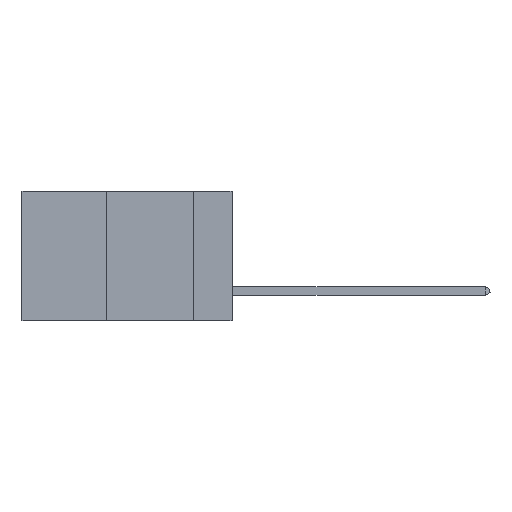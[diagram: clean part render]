
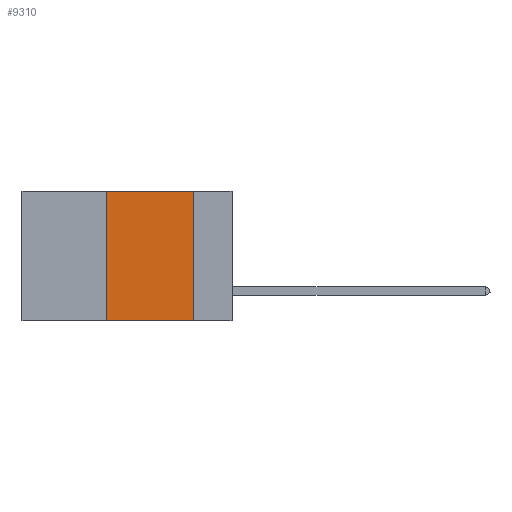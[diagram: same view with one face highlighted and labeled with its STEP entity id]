
A CAD part, left-side view. The second image highlights one B-rep face of the part: STEP entity #9310.
In plain terms, the highlighted planar face has unit normal (-1, 0, 0).
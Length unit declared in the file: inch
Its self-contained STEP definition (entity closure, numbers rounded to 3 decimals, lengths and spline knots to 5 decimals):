
#236 = DIRECTION ( 'NONE',  ( 1., 0., 0. ) ) ;
#335 = AXIS2_PLACEMENT_3D ( 'NONE', #10226, #236, #2248 ) ;
#501 = VERTEX_POINT ( 'NONE', #17729 ) ;
#902 = CARTESIAN_POINT ( 'NONE',  ( 0., 0.11, -0.37 ) ) ;
#1145 = CARTESIAN_POINT ( 'NONE',  ( 0., 0.36, -0.37 ) ) ;
#1899 = LINE ( 'NONE', #17374, #22249 ) ;
#2248 = DIRECTION ( 'NONE',  ( 0., 0., -1. ) ) ;
#3973 = LINE ( 'NONE', #12220, #23406 ) ;
#4230 = EDGE_CURVE ( 'NONE', #18949, #501, #1899, .T. ) ;
#6021 = ORIENTED_EDGE ( 'NONE', *, *, #4230, .F. ) ;
#7247 = VERTEX_POINT ( 'NONE', #902 ) ;
#8017 = DIRECTION ( 'NONE',  ( 0., -1., 0. ) ) ;
#8353 = VECTOR ( 'NONE', #23503, 39.37008 ) ;
#8585 = VERTEX_POINT ( 'NONE', #19391 ) ;
#8626 = EDGE_CURVE ( 'NONE', #8585, #7247, #17283, .T. ) ;
#9310 = ADVANCED_FACE ( 'NONE', ( #23711 ), #13885, .F. ) ;
#10226 = CARTESIAN_POINT ( 'NONE',  ( 0., 0.6, 0. ) ) ;
#12220 = CARTESIAN_POINT ( 'NONE',  ( 0., 0.6, 0. ) ) ;
#13223 = ORIENTED_EDGE ( 'NONE', *, *, #13573, .F. ) ;
#13573 = EDGE_CURVE ( 'NONE', #501, #8585, #3973, .T. ) ;
#13885 = PLANE ( 'NONE',  #335 ) ;
#15218 = DIRECTION ( 'NONE',  ( 0., 0., 1. ) ) ;
#15726 = CARTESIAN_POINT ( 'NONE',  ( 0., 0.6, -0.37 ) ) ;
#15747 = VECTOR ( 'NONE', #18908, 39.37008 ) ;
#17283 = LINE ( 'NONE', #21699, #8353 ) ;
#17374 = CARTESIAN_POINT ( 'NONE',  ( 0., 0.36, 0. ) ) ;
#17729 = CARTESIAN_POINT ( 'NONE',  ( 0., 0.36, 0. ) ) ;
#18055 = EDGE_LOOP ( 'NONE', ( #23101, #13223, #6021, #18713 ) ) ;
#18713 = ORIENTED_EDGE ( 'NONE', *, *, #19095, .T. ) ;
#18908 = DIRECTION ( 'NONE',  ( 0., -1., 0. ) ) ;
#18949 = VERTEX_POINT ( 'NONE', #1145 ) ;
#19095 = EDGE_CURVE ( 'NONE', #18949, #7247, #23744, .T. ) ;
#19391 = CARTESIAN_POINT ( 'NONE',  ( 0., 0.11, 0. ) ) ;
#21699 = CARTESIAN_POINT ( 'NONE',  ( 0., 0.11, 0. ) ) ;
#22249 = VECTOR ( 'NONE', #15218, 39.37008 ) ;
#23101 = ORIENTED_EDGE ( 'NONE', *, *, #8626, .F. ) ;
#23406 = VECTOR ( 'NONE', #8017, 39.37008 ) ;
#23503 = DIRECTION ( 'NONE',  ( 0., 0., -1. ) ) ;
#23711 = FACE_OUTER_BOUND ( 'NONE', #18055, .T. ) ;
#23744 = LINE ( 'NONE', #15726, #15747 ) ;
